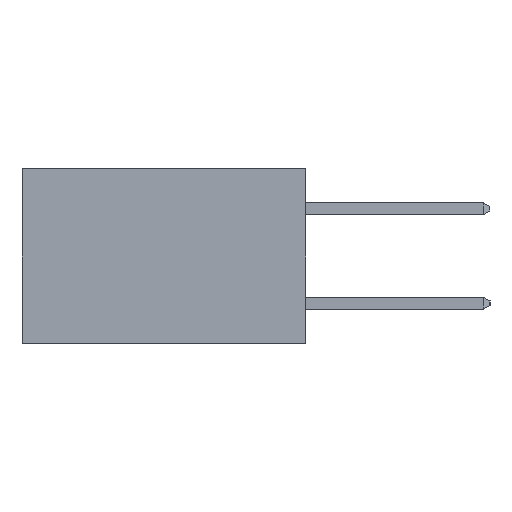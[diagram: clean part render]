
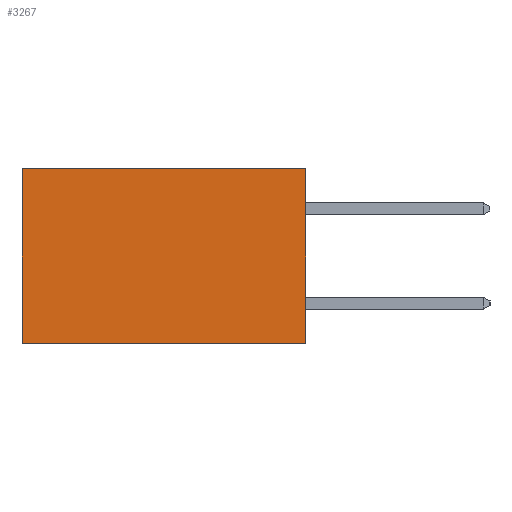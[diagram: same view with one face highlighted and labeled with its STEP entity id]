
A CAD part, left-side view. The second image highlights one B-rep face of the part: STEP entity #3267.
In plain terms, the highlighted planar face has unit normal (-1, 0, 0).
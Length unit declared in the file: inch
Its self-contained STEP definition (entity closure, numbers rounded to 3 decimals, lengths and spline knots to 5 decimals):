
#287 = CARTESIAN_POINT ( 'NONE',  ( 0.2615, 0., 0. ) ) ;
#1368 = ORIENTED_EDGE ( 'NONE', *, *, #10319, .F. ) ;
#2040 = ORIENTED_EDGE ( 'NONE', *, *, #9075, .T. ) ;
#2455 = LINE ( 'NONE', #287, #8321 ) ;
#3267 = ADVANCED_FACE ( 'NONE', ( #21992 ), #11766, .F. ) ;
#3967 = AXIS2_PLACEMENT_3D ( 'NONE', #11704, #11524, #11440 ) ;
#4331 = DIRECTION ( 'NONE',  ( 0., 1., 0. ) ) ;
#4777 = VECTOR ( 'NONE', #11979, 39.37008 ) ;
#5491 = VECTOR ( 'NONE', #25149, 39.37008 ) ;
#8008 = ORIENTED_EDGE ( 'NONE', *, *, #15627, .T. ) ;
#8321 = VECTOR ( 'NONE', #4331, 39.37008 ) ;
#8881 = VERTEX_POINT ( 'NONE', #20786 ) ;
#9075 = EDGE_CURVE ( 'NONE', #13933, #8881, #23767, .T. ) ;
#9174 = CARTESIAN_POINT ( 'NONE',  ( 0.2615, 0., 0. ) ) ;
#10025 = CARTESIAN_POINT ( 'NONE',  ( 0.2615, 0., -0.37 ) ) ;
#10319 = EDGE_CURVE ( 'NONE', #15254, #20639, #15943, .T. ) ;
#11440 = DIRECTION ( 'NONE',  ( 0., 0., -1. ) ) ;
#11524 = DIRECTION ( 'NONE',  ( 1., 0., 0. ) ) ;
#11704 = CARTESIAN_POINT ( 'NONE',  ( 0.2615, 0., -0.37 ) ) ;
#11766 = PLANE ( 'NONE',  #3967 ) ;
#11979 = DIRECTION ( 'NONE',  ( 0., 1., 0. ) ) ;
#12952 = VECTOR ( 'NONE', #13234, 39.37008 ) ;
#13234 = DIRECTION ( 'NONE',  ( 0., 0., -1. ) ) ;
#13933 = VERTEX_POINT ( 'NONE', #20826 ) ;
#14252 = ORIENTED_EDGE ( 'NONE', *, *, #25165, .F. ) ;
#15118 = EDGE_LOOP ( 'NONE', ( #2040, #14252, #1368, #8008 ) ) ;
#15254 = VERTEX_POINT ( 'NONE', #9174 ) ;
#15546 = CARTESIAN_POINT ( 'NONE',  ( 0.2615, 0.6, -0.37 ) ) ;
#15627 = EDGE_CURVE ( 'NONE', #15254, #13933, #2455, .T. ) ;
#15943 = LINE ( 'NONE', #23246, #5491 ) ;
#17567 = CARTESIAN_POINT ( 'NONE',  ( 0.2615, 0., -0.37 ) ) ;
#20309 = LINE ( 'NONE', #10025, #4777 ) ;
#20639 = VERTEX_POINT ( 'NONE', #17567 ) ;
#20786 = CARTESIAN_POINT ( 'NONE',  ( 0.2615, 0.6, -0.37 ) ) ;
#20826 = CARTESIAN_POINT ( 'NONE',  ( 0.2615, 0.6, 0. ) ) ;
#21992 = FACE_OUTER_BOUND ( 'NONE', #15118, .T. ) ;
#23246 = CARTESIAN_POINT ( 'NONE',  ( 0.2615, 0., -0.37 ) ) ;
#23767 = LINE ( 'NONE', #15546, #12952 ) ;
#25149 = DIRECTION ( 'NONE',  ( 0., 0., -1. ) ) ;
#25165 = EDGE_CURVE ( 'NONE', #20639, #8881, #20309, .T. ) ;
